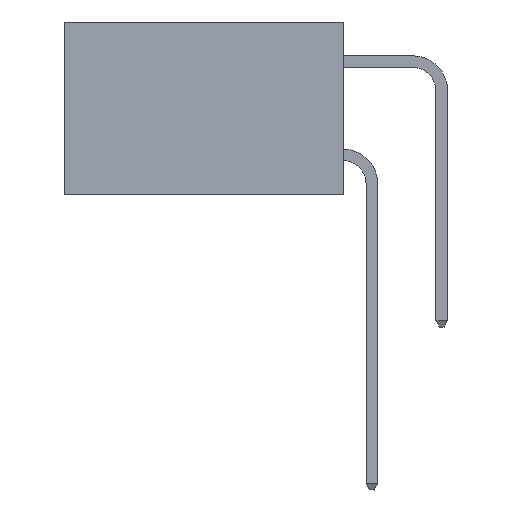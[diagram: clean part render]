
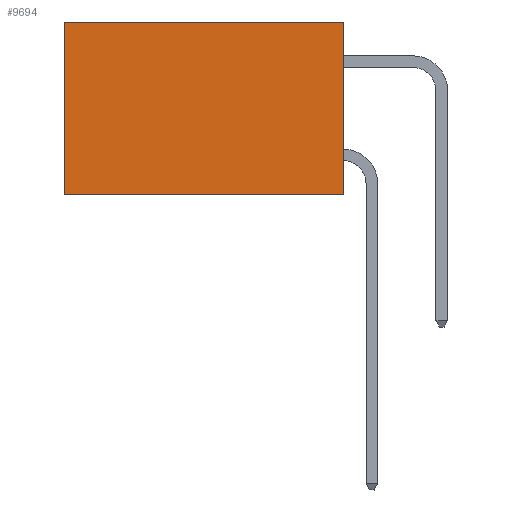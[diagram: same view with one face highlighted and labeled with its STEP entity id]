
A CAD part, left-side view. The second image highlights one B-rep face of the part: STEP entity #9694.
In plain terms, the highlighted planar face has unit normal (-1, 0, 0).
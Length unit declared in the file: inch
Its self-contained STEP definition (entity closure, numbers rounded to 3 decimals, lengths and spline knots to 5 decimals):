
#337 = ORIENTED_EDGE ( 'NONE', *, *, #15127, .F. ) ;
#1435 = DIRECTION ( 'NONE',  ( 0., 0., -1. ) ) ;
#1577 = VERTEX_POINT ( 'NONE', #18819 ) ;
#3061 = VECTOR ( 'NONE', #1435, 39.37008 ) ;
#3089 = CARTESIAN_POINT ( 'NONE',  ( 0.298, 0., 0. ) ) ;
#3430 = AXIS2_PLACEMENT_3D ( 'NONE', #15318, #6140, #16808 ) ;
#3801 = VECTOR ( 'NONE', #4714, 39.37008 ) ;
#4714 = DIRECTION ( 'NONE',  ( 0., 0., -1. ) ) ;
#5145 = VERTEX_POINT ( 'NONE', #8216 ) ;
#5758 = CARTESIAN_POINT ( 'NONE',  ( 0.298, 0.6, 0. ) ) ;
#6140 = DIRECTION ( 'NONE',  ( 1., 0., 0. ) ) ;
#6171 = CARTESIAN_POINT ( 'NONE',  ( 0.298, 0.6, -0.37 ) ) ;
#6454 = ORIENTED_EDGE ( 'NONE', *, *, #14490, .T. ) ;
#6726 = VERTEX_POINT ( 'NONE', #6171 ) ;
#7134 = DIRECTION ( 'NONE',  ( 0., 1., 0. ) ) ;
#7807 = EDGE_CURVE ( 'NONE', #5145, #12508, #10817, .T. ) ;
#8216 = CARTESIAN_POINT ( 'NONE',  ( 0.298, 0., 0. ) ) ;
#8619 = EDGE_LOOP ( 'NONE', ( #6454, #14779, #337, #18080 ) ) ;
#9290 = CARTESIAN_POINT ( 'NONE',  ( 0.298, 0.6, 0. ) ) ;
#9551 = LINE ( 'NONE', #15729, #16652 ) ;
#9694 = ADVANCED_FACE ( 'NONE', ( #10491 ), #16752, .F. ) ;
#10491 = FACE_OUTER_BOUND ( 'NONE', #8619, .T. ) ;
#10817 = LINE ( 'NONE', #16276, #14371 ) ;
#12044 = LINE ( 'NONE', #3089, #3801 ) ;
#12508 = VERTEX_POINT ( 'NONE', #5758 ) ;
#12754 = DIRECTION ( 'NONE',  ( 0., 1., 0. ) ) ;
#14371 = VECTOR ( 'NONE', #7134, 39.37008 ) ;
#14490 = EDGE_CURVE ( 'NONE', #12508, #6726, #19333, .T. ) ;
#14779 = ORIENTED_EDGE ( 'NONE', *, *, #17763, .F. ) ;
#15127 = EDGE_CURVE ( 'NONE', #5145, #1577, #12044, .T. ) ;
#15318 = CARTESIAN_POINT ( 'NONE',  ( 0.298, 0., 0. ) ) ;
#15729 = CARTESIAN_POINT ( 'NONE',  ( 0.298, 0., -0.37 ) ) ;
#16276 = CARTESIAN_POINT ( 'NONE',  ( 0.298, 0., 0. ) ) ;
#16652 = VECTOR ( 'NONE', #12754, 39.37008 ) ;
#16752 = PLANE ( 'NONE',  #3430 ) ;
#16808 = DIRECTION ( 'NONE',  ( 0., 0., -1. ) ) ;
#17763 = EDGE_CURVE ( 'NONE', #1577, #6726, #9551, .T. ) ;
#18080 = ORIENTED_EDGE ( 'NONE', *, *, #7807, .T. ) ;
#18819 = CARTESIAN_POINT ( 'NONE',  ( 0.298, 0., -0.37 ) ) ;
#19333 = LINE ( 'NONE', #9290, #3061 ) ;
